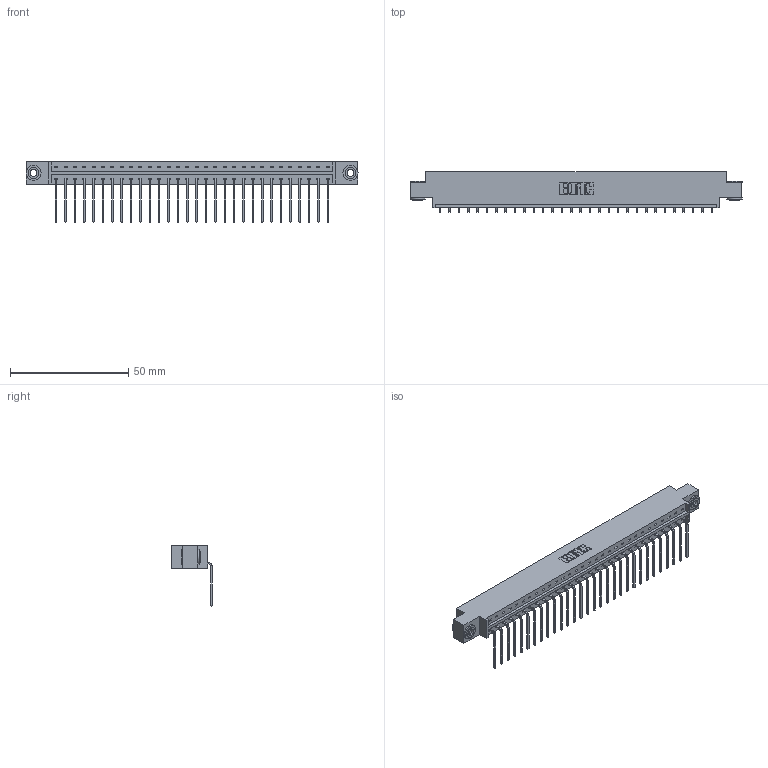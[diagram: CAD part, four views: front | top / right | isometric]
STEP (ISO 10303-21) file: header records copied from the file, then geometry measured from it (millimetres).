
FILE_DESCRIPTION (( 'STEP AP203' ), '1' );
FILE_NAME ('333-030-559-603.STEP', '2018-08-02T19:00:15', ( '' ), ( '' ), 'SwSTEP 2.0', 'SolidWorks 2016', '' );
FILE_SCHEMA (( 'CONFIG_CONTROL_DESIGN' ));
Length unit declared in the file: inch
Products named in the file (4): 333 Part_Offset - .156 Dia - TH; 345-292-001_558 559 Tail - 1; 345-250-002_345-250-002-102; 333-030-559-603
Assembly tree (33 placements, depth 2):
  333-030-559-603
    333 Part_Offset - .156 Dia - TH
    345-292-001_558 559 Tail - 1  x30
    345-250-002_345-250-002-102  x2
Bounding box: 140.41 x 17.09 x 25.53 mm (x, y, z)
Volume: 13917.7 mm3; surface area: 16018.7 mm2
Topology: 33 solids, 33 shells, 1956 faces, 5859 edges, 3862 vertices
Faces by surface type: plane 1404, cylinder 544, cone 8
Entity records: 20758 total; most frequent: CARTESIAN_POINT 3563, ORIENTED_EDGE 3522, DIRECTION 3063, EDGE_CURVE 1761, VECTOR 1609, LINE 1609, VERTEX_POINT 1170, AXIS2_PLACEMENT_3D 727
